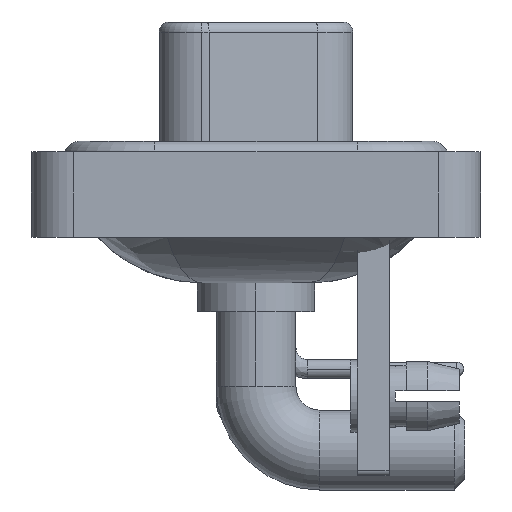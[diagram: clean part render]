
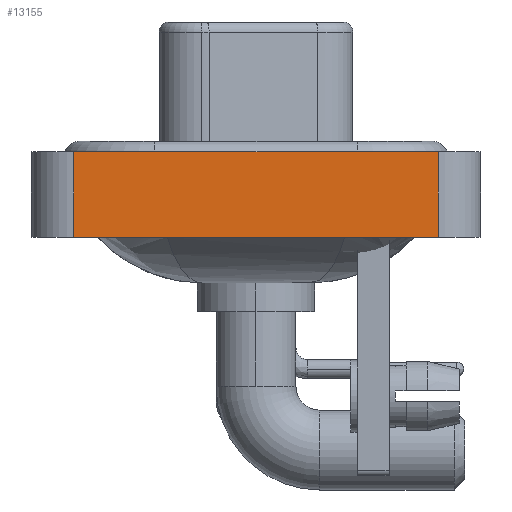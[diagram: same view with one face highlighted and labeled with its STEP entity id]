
A CAD part, left-side view. The second image highlights one B-rep face of the part: STEP entity #13155.
In plain terms, the highlighted planar face has unit normal (-1, 0, 0).
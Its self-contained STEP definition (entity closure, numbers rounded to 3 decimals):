
#247 = LINE ( 'NONE', #18014, #11954 ) ;
#842 = FACE_OUTER_BOUND ( 'NONE', #24812, .T. ) ;
#1249 = CARTESIAN_POINT ( 'NONE',  ( -7.35, 8.55, -3.6 ) ) ;
#1455 = DIRECTION ( 'NONE',  ( 0., -1., 0. ) ) ;
#1600 = ORIENTED_EDGE ( 'NONE', *, *, #17796, .T. ) ;
#1823 = LINE ( 'NONE', #1249, #4564 ) ;
#3030 = LINE ( 'NONE', #9377, #17311 ) ;
#3854 = VERTEX_POINT ( 'NONE', #5872 ) ;
#4564 = VECTOR ( 'NONE', #8452, 1000. ) ;
#5554 = AXIS2_PLACEMENT_3D ( 'NONE', #9352, #25365, #13839 ) ;
#5872 = CARTESIAN_POINT ( 'NONE',  ( -7.35, -8.55, 0.4 ) ) ;
#6843 = VERTEX_POINT ( 'NONE', #20857 ) ;
#8452 = DIRECTION ( 'NONE',  ( 0., 0., 1. ) ) ;
#9352 = CARTESIAN_POINT ( 'NONE',  ( -7.35, -8.55, -3.6 ) ) ;
#9377 = CARTESIAN_POINT ( 'NONE',  ( -7.35, -8.55, -3.6 ) ) ;
#10478 = CARTESIAN_POINT ( 'NONE',  ( -7.35, 8.55, 0.4 ) ) ;
#11280 = VERTEX_POINT ( 'NONE', #10478 ) ;
#11954 = VECTOR ( 'NONE', #26791, 1000. ) ;
#11977 = DIRECTION ( 'NONE',  ( 0., 0., 1. ) ) ;
#13155 = ADVANCED_FACE ( 'NONE', ( #842 ), #16008, .T. ) ;
#13522 = EDGE_CURVE ( 'NONE', #11280, #3854, #247, .T. ) ;
#13839 = DIRECTION ( 'NONE',  ( 0., 0., 1. ) ) ;
#14878 = LINE ( 'NONE', #16755, #27387 ) ;
#15065 = EDGE_CURVE ( 'NONE', #28127, #11280, #1823, .T. ) ;
#16008 = PLANE ( 'NONE',  #5554 ) ;
#16755 = CARTESIAN_POINT ( 'NONE',  ( -7.35, -8.55, -3.6 ) ) ;
#17311 = VECTOR ( 'NONE', #11977, 1000. ) ;
#17796 = EDGE_CURVE ( 'NONE', #6843, #3854, #3030, .T. ) ;
#18014 = CARTESIAN_POINT ( 'NONE',  ( -7.35, -8.55, 0.4 ) ) ;
#19045 = ORIENTED_EDGE ( 'NONE', *, *, #27224, .T. ) ;
#20813 = ORIENTED_EDGE ( 'NONE', *, *, #15065, .F. ) ;
#20857 = CARTESIAN_POINT ( 'NONE',  ( -7.35, -8.55, -3.6 ) ) ;
#22685 = ORIENTED_EDGE ( 'NONE', *, *, #13522, .F. ) ;
#23071 = CARTESIAN_POINT ( 'NONE',  ( -7.35, 8.55, -3.6 ) ) ;
#24812 = EDGE_LOOP ( 'NONE', ( #1600, #22685, #20813, #19045 ) ) ;
#25365 = DIRECTION ( 'NONE',  ( -1., 0., 0. ) ) ;
#26791 = DIRECTION ( 'NONE',  ( 0., -1., 0. ) ) ;
#27224 = EDGE_CURVE ( 'NONE', #28127, #6843, #14878, .T. ) ;
#27387 = VECTOR ( 'NONE', #1455, 1000. ) ;
#28127 = VERTEX_POINT ( 'NONE', #23071 ) ;
